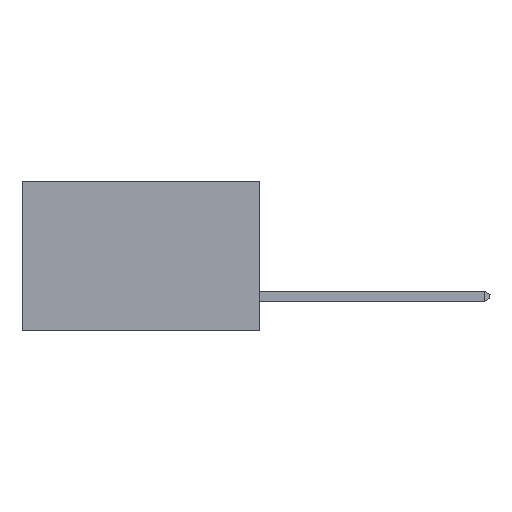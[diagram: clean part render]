
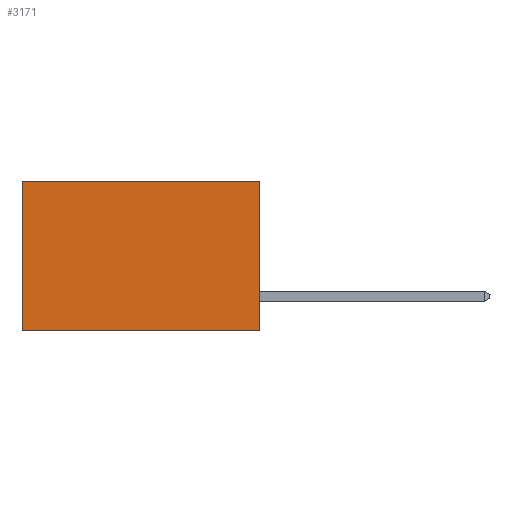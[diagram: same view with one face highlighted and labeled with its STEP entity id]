
A CAD part, left-side view. The second image highlights one B-rep face of the part: STEP entity #3171.
In plain terms, the highlighted planar face has unit normal (-1, 0, 0).
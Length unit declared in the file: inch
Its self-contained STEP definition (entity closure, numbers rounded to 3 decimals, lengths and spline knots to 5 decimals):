
#470 = VECTOR ( 'NONE', #3033, 39.37008 ) ;
#809 = CARTESIAN_POINT ( 'NONE',  ( 0.277, 0., 0. ) ) ;
#967 = DIRECTION ( 'NONE',  ( 0., 1., 0. ) ) ;
#1184 = CARTESIAN_POINT ( 'NONE',  ( 0.277, 0., -0.37 ) ) ;
#1214 = VERTEX_POINT ( 'NONE', #1184 ) ;
#1423 = CARTESIAN_POINT ( 'NONE',  ( 0.277, 0., -0.37 ) ) ;
#1653 = VECTOR ( 'NONE', #967, 39.37008 ) ;
#2041 = EDGE_CURVE ( 'NONE', #1214, #8495, #10192, .T. ) ;
#2057 = EDGE_CURVE ( 'NONE', #3771, #1214, #3731, .T. ) ;
#3033 = DIRECTION ( 'NONE',  ( 0., 0., -1. ) ) ;
#3046 = CARTESIAN_POINT ( 'NONE',  ( 0.277, 0.59, -0.37 ) ) ;
#3171 = ADVANCED_FACE ( 'NONE', ( #4922 ), #5291, .F. ) ;
#3731 = LINE ( 'NONE', #10284, #7663 ) ;
#3771 = VERTEX_POINT ( 'NONE', #5861 ) ;
#3848 = LINE ( 'NONE', #809, #9635 ) ;
#4922 = FACE_OUTER_BOUND ( 'NONE', #5910, .T. ) ;
#5084 = AXIS2_PLACEMENT_3D ( 'NONE', #5365, #5217, #5131 ) ;
#5131 = DIRECTION ( 'NONE',  ( 0., 0., -1. ) ) ;
#5217 = DIRECTION ( 'NONE',  ( 1., 0., 0. ) ) ;
#5286 = EDGE_CURVE ( 'NONE', #6777, #8495, #6470, .T. ) ;
#5291 = PLANE ( 'NONE',  #5084 ) ;
#5365 = CARTESIAN_POINT ( 'NONE',  ( 0.277, 0., -0.37 ) ) ;
#5861 = CARTESIAN_POINT ( 'NONE',  ( 0.277, 0., 0. ) ) ;
#5910 = EDGE_LOOP ( 'NONE', ( #6876, #10063, #9111, #6943 ) ) ;
#6470 = LINE ( 'NONE', #3046, #470 ) ;
#6777 = VERTEX_POINT ( 'NONE', #8860 ) ;
#6780 = EDGE_CURVE ( 'NONE', #3771, #6777, #3848, .T. ) ;
#6876 = ORIENTED_EDGE ( 'NONE', *, *, #5286, .T. ) ;
#6943 = ORIENTED_EDGE ( 'NONE', *, *, #6780, .T. ) ;
#7663 = VECTOR ( 'NONE', #10237, 39.37008 ) ;
#7983 = CARTESIAN_POINT ( 'NONE',  ( 0.277, 0.59, -0.37 ) ) ;
#8495 = VERTEX_POINT ( 'NONE', #7983 ) ;
#8714 = DIRECTION ( 'NONE',  ( 0., 1., 0. ) ) ;
#8860 = CARTESIAN_POINT ( 'NONE',  ( 0.277, 0.59, 0. ) ) ;
#9111 = ORIENTED_EDGE ( 'NONE', *, *, #2057, .F. ) ;
#9635 = VECTOR ( 'NONE', #8714, 39.37008 ) ;
#10063 = ORIENTED_EDGE ( 'NONE', *, *, #2041, .F. ) ;
#10192 = LINE ( 'NONE', #1423, #1653 ) ;
#10237 = DIRECTION ( 'NONE',  ( 0., 0., -1. ) ) ;
#10284 = CARTESIAN_POINT ( 'NONE',  ( 0.277, 0., -0.37 ) ) ;
